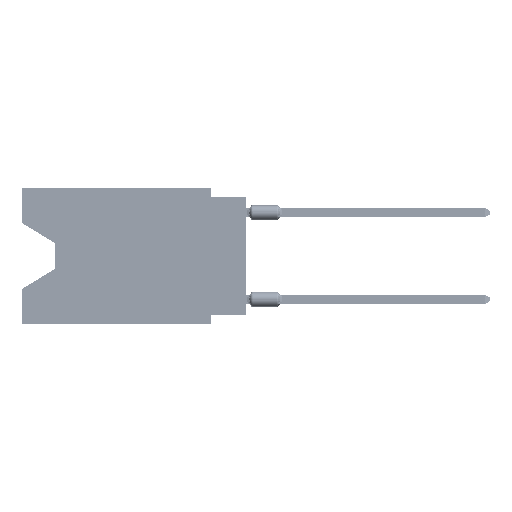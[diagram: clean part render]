
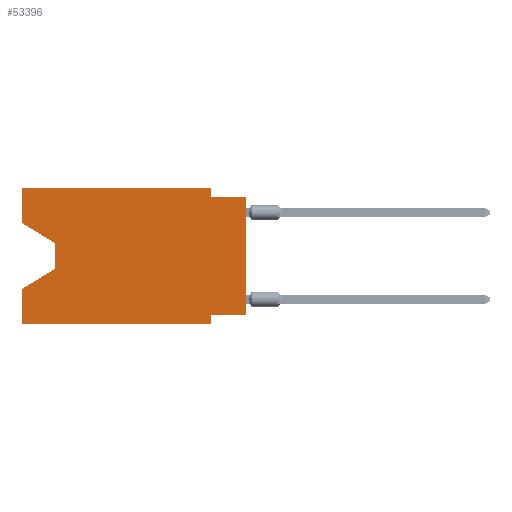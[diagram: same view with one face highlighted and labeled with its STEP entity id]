
A CAD part, left-side view. The second image highlights one B-rep face of the part: STEP entity #53396.
In plain terms, the highlighted planar face has unit normal (-1, 0, 0).
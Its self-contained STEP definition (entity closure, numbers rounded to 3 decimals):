
#466 = DIRECTION ( 'NONE',  ( 0., -1., 0. ) ) ;
#882 = CARTESIAN_POINT ( 'NONE',  ( 0., 0., -0.635 ) ) ;
#1836 = DIRECTION ( 'NONE',  ( 1., 0., 0. ) ) ;
#1847 = ORIENTED_EDGE ( 'NONE', *, *, #69809, .F. ) ;
#2037 = DIRECTION ( 'NONE',  ( 0., -1., 0. ) ) ;
#2288 = LINE ( 'NONE', #37130, #11614 ) ;
#2770 = CARTESIAN_POINT ( 'NONE',  ( 0., 16.383, 0. ) ) ;
#2816 = DIRECTION ( 'NONE',  ( 0., 0., 1. ) ) ;
#3191 = VECTOR ( 'NONE', #61167, 1000. ) ;
#4157 = CARTESIAN_POINT ( 'NONE',  ( 0., 2.54, -9.906 ) ) ;
#5771 = ORIENTED_EDGE ( 'NONE', *, *, #42767, .F. ) ;
#7060 = CARTESIAN_POINT ( 'NONE',  ( 0., 16.383, 0. ) ) ;
#7519 = AXIS2_PLACEMENT_3D ( 'NONE', #7060, #1836, #63365 ) ;
#7639 = DIRECTION ( 'NONE',  ( 0., -0.855, -0.519 ) ) ;
#7786 = VECTOR ( 'NONE', #32940, 1000. ) ;
#8158 = ORIENTED_EDGE ( 'NONE', *, *, #53296, .T. ) ;
#9558 = EDGE_CURVE ( 'NONE', #47784, #59128, #18435, .T. ) ;
#9913 = VECTOR ( 'NONE', #27840, 1000. ) ;
#10220 = VECTOR ( 'NONE', #25711, 1000. ) ;
#10367 = LINE ( 'NONE', #10730, #15994 ) ;
#10730 = CARTESIAN_POINT ( 'NONE',  ( 0., 2.54, -9.906 ) ) ;
#11614 = VECTOR ( 'NONE', #36395, 1000. ) ;
#12349 = LINE ( 'NONE', #23481, #43564 ) ;
#13361 = VERTEX_POINT ( 'NONE', #35632 ) ;
#13416 = VECTOR ( 'NONE', #2816, 1000. ) ;
#14444 = EDGE_CURVE ( 'NONE', #50254, #65821, #50860, .T. ) ;
#15086 = CARTESIAN_POINT ( 'NONE',  ( 0., 16.383, -9.906 ) ) ;
#15690 = EDGE_CURVE ( 'NONE', #48282, #25439, #47674, .T. ) ;
#15994 = VECTOR ( 'NONE', #28129, 1000. ) ;
#16359 = EDGE_LOOP ( 'NONE', ( #39257, #33862, #8158, #23393, #41668, #70495, #56178, #26627, #1847, #23591, #5771, #52185 ) ) ;
#18435 = LINE ( 'NONE', #69540, #10220 ) ;
#19245 = VECTOR ( 'NONE', #61974, 1000. ) ;
#19482 = LINE ( 'NONE', #2770, #50512 ) ;
#20728 = EDGE_CURVE ( 'NONE', #52137, #61207, #43029, .T. ) ;
#21635 = CARTESIAN_POINT ( 'NONE',  ( 0., 16.383, 0. ) ) ;
#22562 = CARTESIAN_POINT ( 'NONE',  ( 0., 0., -9.271 ) ) ;
#22607 = EDGE_CURVE ( 'NONE', #48282, #44415, #28828, .T. ) ;
#23393 = ORIENTED_EDGE ( 'NONE', *, *, #9558, .F. ) ;
#23481 = CARTESIAN_POINT ( 'NONE',  ( 0., 0., -0.635 ) ) ;
#23591 = ORIENTED_EDGE ( 'NONE', *, *, #69910, .F. ) ;
#24404 = CARTESIAN_POINT ( 'NONE',  ( 0., 2.54, -0.635 ) ) ;
#25439 = VERTEX_POINT ( 'NONE', #882 ) ;
#25711 = DIRECTION ( 'NONE',  ( 0., 0., 1. ) ) ;
#25783 = LINE ( 'NONE', #58404, #51954 ) ;
#26627 = ORIENTED_EDGE ( 'NONE', *, *, #15690, .T. ) ;
#26754 = LINE ( 'NONE', #33405, #9913 ) ;
#26851 = CARTESIAN_POINT ( 'NONE',  ( 0., 0., -9.271 ) ) ;
#27840 = DIRECTION ( 'NONE',  ( 0., 0.855, -0.519 ) ) ;
#27996 = VERTEX_POINT ( 'NONE', #4157 ) ;
#28129 = DIRECTION ( 'NONE',  ( 0., 0., -1. ) ) ;
#28828 = LINE ( 'NONE', #22562, #62505 ) ;
#29661 = FACE_OUTER_BOUND ( 'NONE', #16359, .T. ) ;
#32648 = CARTESIAN_POINT ( 'NONE',  ( 0., 13.97, -4.013 ) ) ;
#32940 = DIRECTION ( 'NONE',  ( 0., -1., 0. ) ) ;
#33405 = CARTESIAN_POINT ( 'NONE',  ( 0., 13.97, -5.893 ) ) ;
#33572 = EDGE_CURVE ( 'NONE', #50254, #52137, #25783, .T. ) ;
#33862 = ORIENTED_EDGE ( 'NONE', *, *, #20728, .T. ) ;
#35632 = CARTESIAN_POINT ( 'NONE',  ( 0., 2.54, 0. ) ) ;
#36395 = DIRECTION ( 'NONE',  ( 0., 0., -1. ) ) ;
#37130 = CARTESIAN_POINT ( 'NONE',  ( 0., 2.54, 0. ) ) ;
#39229 = LINE ( 'NONE', #61094, #7786 ) ;
#39257 = ORIENTED_EDGE ( 'NONE', *, *, #33572, .T. ) ;
#41537 = CARTESIAN_POINT ( 'NONE',  ( 0., 16.383, -2.546 ) ) ;
#41668 = ORIENTED_EDGE ( 'NONE', *, *, #69443, .T. ) ;
#42767 = EDGE_CURVE ( 'NONE', #65821, #13361, #19482, .T. ) ;
#43029 = LINE ( 'NONE', #32648, #3191 ) ;
#43564 = VECTOR ( 'NONE', #466, 1000. ) ;
#44415 = VERTEX_POINT ( 'NONE', #60120 ) ;
#45081 = CARTESIAN_POINT ( 'NONE',  ( 0., 16.383, 0. ) ) ;
#46243 = DIRECTION ( 'NONE',  ( 0., 1., 0. ) ) ;
#47674 = LINE ( 'NONE', #53601, #13416 ) ;
#47784 = VERTEX_POINT ( 'NONE', #15086 ) ;
#48282 = VERTEX_POINT ( 'NONE', #26851 ) ;
#50254 = VERTEX_POINT ( 'NONE', #41537 ) ;
#50512 = VECTOR ( 'NONE', #2037, 1000. ) ;
#50860 = LINE ( 'NONE', #21635, #19245 ) ;
#51954 = VECTOR ( 'NONE', #7639, 1000. ) ;
#52137 = VERTEX_POINT ( 'NONE', #60830 ) ;
#52185 = ORIENTED_EDGE ( 'NONE', *, *, #14444, .F. ) ;
#53296 = EDGE_CURVE ( 'NONE', #61207, #59128, #26754, .T. ) ;
#53396 = ADVANCED_FACE ( 'NONE', ( #29661 ), #63006, .F. ) ;
#53601 = CARTESIAN_POINT ( 'NONE',  ( 0., 0., 0. ) ) ;
#54928 = EDGE_CURVE ( 'NONE', #44415, #27996, #10367, .T. ) ;
#56178 = ORIENTED_EDGE ( 'NONE', *, *, #22607, .F. ) ;
#57331 = CARTESIAN_POINT ( 'NONE',  ( 0., 16.383, -7.36 ) ) ;
#57555 = VERTEX_POINT ( 'NONE', #24404 ) ;
#58404 = CARTESIAN_POINT ( 'NONE',  ( 0., 16.383, -2.546 ) ) ;
#58470 = CARTESIAN_POINT ( 'NONE',  ( 0., 13.97, -5.893 ) ) ;
#59128 = VERTEX_POINT ( 'NONE', #57331 ) ;
#60120 = CARTESIAN_POINT ( 'NONE',  ( 0., 2.54, -9.271 ) ) ;
#60830 = CARTESIAN_POINT ( 'NONE',  ( 0., 13.97, -4.013 ) ) ;
#61094 = CARTESIAN_POINT ( 'NONE',  ( 0., 16.383, -9.906 ) ) ;
#61167 = DIRECTION ( 'NONE',  ( 0., 0., -1. ) ) ;
#61207 = VERTEX_POINT ( 'NONE', #58470 ) ;
#61974 = DIRECTION ( 'NONE',  ( 0., 0., 1. ) ) ;
#62505 = VECTOR ( 'NONE', #46243, 1000. ) ;
#63006 = PLANE ( 'NONE',  #7519 ) ;
#63365 = DIRECTION ( 'NONE',  ( 0., 0., -1. ) ) ;
#65821 = VERTEX_POINT ( 'NONE', #45081 ) ;
#69443 = EDGE_CURVE ( 'NONE', #47784, #27996, #39229, .T. ) ;
#69540 = CARTESIAN_POINT ( 'NONE',  ( 0., 16.383, 0. ) ) ;
#69809 = EDGE_CURVE ( 'NONE', #57555, #25439, #12349, .T. ) ;
#69910 = EDGE_CURVE ( 'NONE', #13361, #57555, #2288, .T. ) ;
#70495 = ORIENTED_EDGE ( 'NONE', *, *, #54928, .F. ) ;
